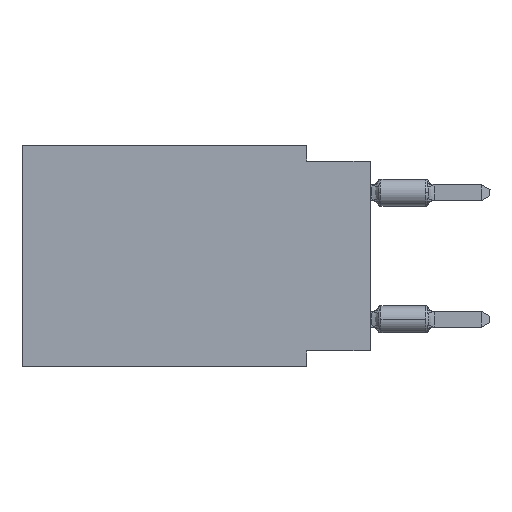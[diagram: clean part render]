
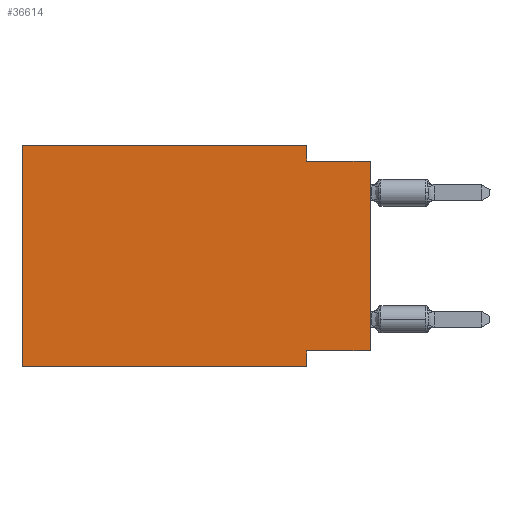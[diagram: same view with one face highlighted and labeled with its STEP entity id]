
A CAD part, left-side view. The second image highlights one B-rep face of the part: STEP entity #36614.
In plain terms, the highlighted planar face has unit normal (-1, 0, 0).
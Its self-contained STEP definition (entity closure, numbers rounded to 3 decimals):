
#471 = LINE ( 'NONE', #45602, #44120 ) ;
#1843 = CARTESIAN_POINT ( 'NONE',  ( 0., 13.97, -8.89 ) ) ;
#2055 = VERTEX_POINT ( 'NONE', #41671 ) ;
#5615 = CARTESIAN_POINT ( 'NONE',  ( 0., 2.54, -8.255 ) ) ;
#5750 = LINE ( 'NONE', #42418, #45982 ) ;
#5940 = EDGE_CURVE ( 'NONE', #31279, #2055, #471, .T. ) ;
#5956 = LINE ( 'NONE', #14644, #45861 ) ;
#6192 = ORIENTED_EDGE ( 'NONE', *, *, #5940, .F. ) ;
#6971 = CARTESIAN_POINT ( 'NONE',  ( 0., 13.97, -8.89 ) ) ;
#7195 = CARTESIAN_POINT ( 'NONE',  ( 0., 0., -0.635 ) ) ;
#7405 = CARTESIAN_POINT ( 'NONE',  ( 0., 0., -8.255 ) ) ;
#8004 = LINE ( 'NONE', #53398, #21490 ) ;
#9084 = CARTESIAN_POINT ( 'NONE',  ( 0., 0., -0.635 ) ) ;
#10900 = VERTEX_POINT ( 'NONE', #7195 ) ;
#11243 = ORIENTED_EDGE ( 'NONE', *, *, #27835, .T. ) ;
#11663 = FACE_OUTER_BOUND ( 'NONE', #50269, .T. ) ;
#11964 = DIRECTION ( 'NONE',  ( 0., 0., -1. ) ) ;
#12561 = CARTESIAN_POINT ( 'NONE',  ( 0., 13.97, 0. ) ) ;
#14644 = CARTESIAN_POINT ( 'NONE',  ( 0., 13.97, 0. ) ) ;
#14946 = VERTEX_POINT ( 'NONE', #51613 ) ;
#15052 = CARTESIAN_POINT ( 'NONE',  ( 0., 13.97, 0. ) ) ;
#15066 = VERTEX_POINT ( 'NONE', #7405 ) ;
#17127 = EDGE_CURVE ( 'NONE', #23255, #55283, #8004, .T. ) ;
#17824 = EDGE_CURVE ( 'NONE', #45956, #14946, #52071, .T. ) ;
#20045 = VECTOR ( 'NONE', #24826, 1000. ) ;
#20150 = DIRECTION ( 'NONE',  ( 0., -1., 0. ) ) ;
#20350 = DIRECTION ( 'NONE',  ( 0., -1., 0. ) ) ;
#21490 = VECTOR ( 'NONE', #35654, 1000. ) ;
#23255 = VERTEX_POINT ( 'NONE', #5615 ) ;
#24826 = DIRECTION ( 'NONE',  ( 0., 1., 0. ) ) ;
#27835 = EDGE_CURVE ( 'NONE', #45956, #55283, #56839, .T. ) ;
#28748 = ORIENTED_EDGE ( 'NONE', *, *, #17824, .F. ) ;
#29950 = ORIENTED_EDGE ( 'NONE', *, *, #17127, .F. ) ;
#31279 = VERTEX_POINT ( 'NONE', #58407 ) ;
#31353 = VECTOR ( 'NONE', #55086, 1000. ) ;
#34009 = DIRECTION ( 'NONE',  ( 0., 0., 1. ) ) ;
#35654 = DIRECTION ( 'NONE',  ( 0., 0., -1. ) ) ;
#36614 = ADVANCED_FACE ( 'NONE', ( #11663 ), #52867, .F. ) ;
#37769 = ORIENTED_EDGE ( 'NONE', *, *, #44526, .F. ) ;
#38304 = EDGE_CURVE ( 'NONE', #15066, #23255, #51593, .T. ) ;
#38428 = ORIENTED_EDGE ( 'NONE', *, *, #38304, .F. ) ;
#41074 = DIRECTION ( 'NONE',  ( 0., 0., -1. ) ) ;
#41611 = CARTESIAN_POINT ( 'NONE',  ( 0., 2.54, -8.89 ) ) ;
#41671 = CARTESIAN_POINT ( 'NONE',  ( 0., 2.54, -0.635 ) ) ;
#41752 = ORIENTED_EDGE ( 'NONE', *, *, #54136, .T. ) ;
#42418 = CARTESIAN_POINT ( 'NONE',  ( 0., 0., 0. ) ) ;
#42716 = DIRECTION ( 'NONE',  ( 0., 0., 1. ) ) ;
#43545 = DIRECTION ( 'NONE',  ( 1., 0., 0. ) ) ;
#43951 = AXIS2_PLACEMENT_3D ( 'NONE', #12561, #43545, #11964 ) ;
#44120 = VECTOR ( 'NONE', #41074, 1000. ) ;
#44144 = ORIENTED_EDGE ( 'NONE', *, *, #53382, .F. ) ;
#44526 = EDGE_CURVE ( 'NONE', #2055, #10900, #50575, .T. ) ;
#45602 = CARTESIAN_POINT ( 'NONE',  ( 0., 2.54, 0. ) ) ;
#45861 = VECTOR ( 'NONE', #20350, 1000. ) ;
#45956 = VERTEX_POINT ( 'NONE', #6971 ) ;
#45982 = VECTOR ( 'NONE', #42716, 1000. ) ;
#50269 = EDGE_LOOP ( 'NONE', ( #41752, #37769, #6192, #44144, #28748, #11243, #29950, #38428 ) ) ;
#50330 = VECTOR ( 'NONE', #34009, 1000. ) ;
#50575 = LINE ( 'NONE', #9084, #31353 ) ;
#51593 = LINE ( 'NONE', #56994, #20045 ) ;
#51613 = CARTESIAN_POINT ( 'NONE',  ( 0., 13.97, 0. ) ) ;
#52071 = LINE ( 'NONE', #15052, #50330 ) ;
#52867 = PLANE ( 'NONE',  #43951 ) ;
#53382 = EDGE_CURVE ( 'NONE', #14946, #31279, #5956, .T. ) ;
#53398 = CARTESIAN_POINT ( 'NONE',  ( 0., 2.54, -8.89 ) ) ;
#54136 = EDGE_CURVE ( 'NONE', #15066, #10900, #5750, .T. ) ;
#55086 = DIRECTION ( 'NONE',  ( 0., -1., 0. ) ) ;
#55283 = VERTEX_POINT ( 'NONE', #41611 ) ;
#56839 = LINE ( 'NONE', #1843, #57700 ) ;
#56994 = CARTESIAN_POINT ( 'NONE',  ( 0., 0., -8.255 ) ) ;
#57700 = VECTOR ( 'NONE', #20150, 1000. ) ;
#58407 = CARTESIAN_POINT ( 'NONE',  ( 0., 2.54, 0. ) ) ;
